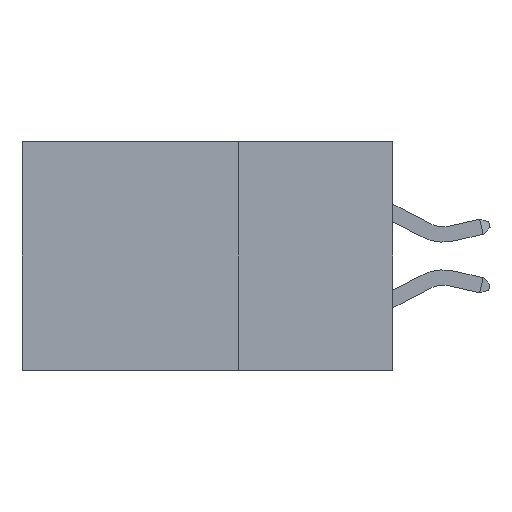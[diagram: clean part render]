
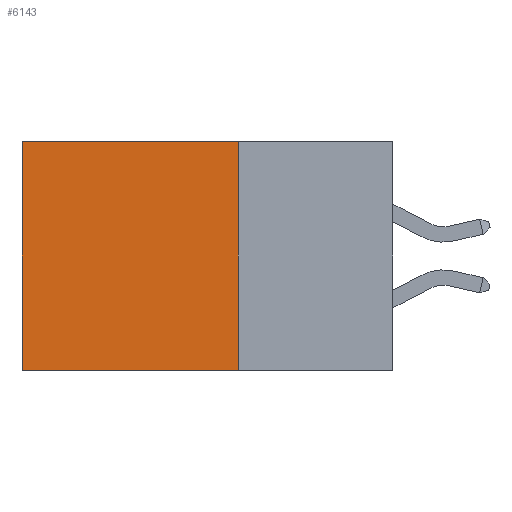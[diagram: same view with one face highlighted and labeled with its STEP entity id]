
A CAD part, left-side view. The second image highlights one B-rep face of the part: STEP entity #6143.
In plain terms, the highlighted planar face has unit normal (-1, 0, 0).
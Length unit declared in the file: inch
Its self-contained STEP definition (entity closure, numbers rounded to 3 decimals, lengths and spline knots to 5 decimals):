
#299 = CARTESIAN_POINT ( 'NONE',  ( 0.2875, 0.6, 0. ) ) ;
#586 = DIRECTION ( 'NONE',  ( 0., 1., 0. ) ) ;
#1443 = PLANE ( 'NONE',  #21796 ) ;
#2083 = CARTESIAN_POINT ( 'NONE',  ( 0.2875, 0.25, -0.37 ) ) ;
#2213 = VERTEX_POINT ( 'NONE', #299 ) ;
#2484 = EDGE_LOOP ( 'NONE', ( #23808, #23733, #15638, #4550 ) ) ;
#2491 = LINE ( 'NONE', #13016, #7779 ) ;
#2547 = VECTOR ( 'NONE', #21564, 39.37008 ) ;
#3467 = DIRECTION ( 'NONE',  ( 1., 0., 0. ) ) ;
#3477 = EDGE_CURVE ( 'NONE', #11788, #3718, #4879, .T. ) ;
#3718 = VERTEX_POINT ( 'NONE', #5064 ) ;
#4550 = ORIENTED_EDGE ( 'NONE', *, *, #16314, .T. ) ;
#4879 = LINE ( 'NONE', #14276, #20209 ) ;
#5064 = CARTESIAN_POINT ( 'NONE',  ( 0.2875, 0.6, -0.37 ) ) ;
#6143 = ADVANCED_FACE ( 'NONE', ( #9408 ), #1443, .F. ) ;
#7779 = VECTOR ( 'NONE', #19031, 39.37008 ) ;
#7800 = VERTEX_POINT ( 'NONE', #13321 ) ;
#8367 = EDGE_CURVE ( 'NONE', #7800, #11788, #2491, .T. ) ;
#9373 = CARTESIAN_POINT ( 'NONE',  ( 0.2875, 0.25, 0. ) ) ;
#9408 = FACE_OUTER_BOUND ( 'NONE', #2484, .T. ) ;
#10545 = CARTESIAN_POINT ( 'NONE',  ( 0.2875, 0.25, 0. ) ) ;
#11572 = CARTESIAN_POINT ( 'NONE',  ( 0.2875, 0.6, 0. ) ) ;
#11788 = VERTEX_POINT ( 'NONE', #2083 ) ;
#13016 = CARTESIAN_POINT ( 'NONE',  ( 0.2875, 0.25, 0. ) ) ;
#13133 = EDGE_CURVE ( 'NONE', #2213, #3718, #18468, .T. ) ;
#13321 = CARTESIAN_POINT ( 'NONE',  ( 0.2875, 0.25, 0. ) ) ;
#13805 = VECTOR ( 'NONE', #586, 39.37008 ) ;
#14276 = CARTESIAN_POINT ( 'NONE',  ( 0.2875, 0.25, -0.37 ) ) ;
#15638 = ORIENTED_EDGE ( 'NONE', *, *, #8367, .F. ) ;
#16314 = EDGE_CURVE ( 'NONE', #7800, #2213, #18458, .T. ) ;
#17439 = DIRECTION ( 'NONE',  ( 0., 0., -1. ) ) ;
#18458 = LINE ( 'NONE', #10545, #13805 ) ;
#18468 = LINE ( 'NONE', #11572, #2547 ) ;
#19031 = DIRECTION ( 'NONE',  ( 0., 0., -1. ) ) ;
#20209 = VECTOR ( 'NONE', #24284, 39.37008 ) ;
#21564 = DIRECTION ( 'NONE',  ( 0., 0., -1. ) ) ;
#21796 = AXIS2_PLACEMENT_3D ( 'NONE', #9373, #3467, #17439 ) ;
#23733 = ORIENTED_EDGE ( 'NONE', *, *, #3477, .F. ) ;
#23808 = ORIENTED_EDGE ( 'NONE', *, *, #13133, .T. ) ;
#24284 = DIRECTION ( 'NONE',  ( 0., 1., 0. ) ) ;
